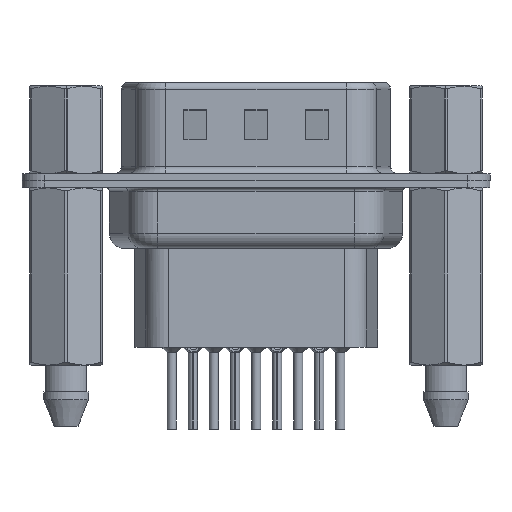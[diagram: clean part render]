
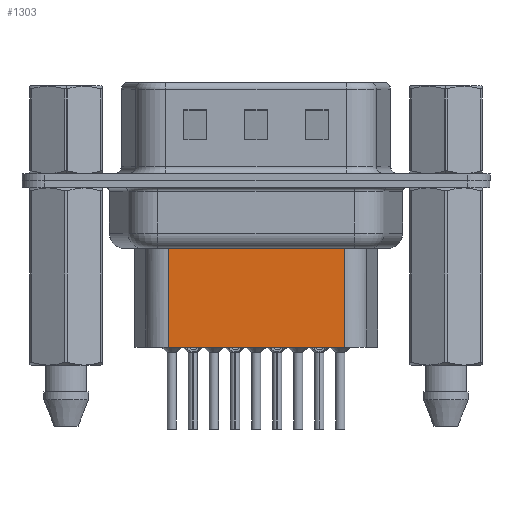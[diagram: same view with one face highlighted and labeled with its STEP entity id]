
A CAD part, front view. The second image highlights one B-rep face of the part: STEP entity #1303.
In plain terms, the highlighted planar face has unit normal (0, -1, 0).
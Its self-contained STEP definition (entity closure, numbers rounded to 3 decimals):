
#412 = DIRECTION ( 'NONE',  ( -1., 0., 0. ) ) ;
#484 = LINE ( 'NONE', #8656, #5251 ) ;
#1233 = VECTOR ( 'NONE', #412, 1000. ) ;
#1303 = ADVANCED_FACE ( 'NONE', ( #20888 ), #2808, .T. ) ;
#1419 = AXIS2_PLACEMENT_3D ( 'NONE', #17182, #10884, #6892 ) ;
#1904 = VECTOR ( 'NONE', #1964, 1000. ) ;
#1964 = DIRECTION ( 'NONE',  ( 0., 0., -1. ) ) ;
#2642 = VERTEX_POINT ( 'NONE', #18498 ) ;
#2776 = ORIENTED_EDGE ( 'NONE', *, *, #24345, .T. ) ;
#2808 = PLANE ( 'NONE',  #1419 ) ;
#3517 = LINE ( 'NONE', #9584, #23152 ) ;
#4767 = ORIENTED_EDGE ( 'NONE', *, *, #11726, .F. ) ;
#5251 = VECTOR ( 'NONE', #14595, 1000. ) ;
#5622 = DIRECTION ( 'NONE',  ( -1., 0., 0. ) ) ;
#6504 = EDGE_LOOP ( 'NONE', ( #4767, #2776, #11602, #25005 ) ) ;
#6892 = DIRECTION ( 'NONE',  ( 1., 0., 0. ) ) ;
#6987 = LINE ( 'NONE', #18492, #1233 ) ;
#7474 = VERTEX_POINT ( 'NONE', #15951 ) ;
#7946 = VERTEX_POINT ( 'NONE', #21396 ) ;
#8275 = CARTESIAN_POINT ( 'NONE',  ( 6.706, -3.5, -10.95 ) ) ;
#8656 = CARTESIAN_POINT ( 'NONE',  ( 6.706, -3.5, -3.1 ) ) ;
#9584 = CARTESIAN_POINT ( 'NONE',  ( 6.459, -3.5, -4.097 ) ) ;
#10884 = DIRECTION ( 'NONE',  ( 0., -1., 0. ) ) ;
#10988 = EDGE_CURVE ( 'NONE', #2642, #19853, #484, .T. ) ;
#11602 = ORIENTED_EDGE ( 'NONE', *, *, #10988, .T. ) ;
#11726 = EDGE_CURVE ( 'NONE', #7474, #7946, #25851, .T. ) ;
#14595 = DIRECTION ( 'NONE',  ( 0., 0., -1. ) ) ;
#15951 = CARTESIAN_POINT ( 'NONE',  ( 18.294, -3.5, -4.097 ) ) ;
#17182 = CARTESIAN_POINT ( 'NONE',  ( 6.706, -3.5, -3.1 ) ) ;
#18492 = CARTESIAN_POINT ( 'NONE',  ( 6.706, -3.5, -10.95 ) ) ;
#18498 = CARTESIAN_POINT ( 'NONE',  ( 6.706, -3.5, -4.097 ) ) ;
#19853 = VERTEX_POINT ( 'NONE', #8275 ) ;
#20888 = FACE_OUTER_BOUND ( 'NONE', #6504, .T. ) ;
#21396 = CARTESIAN_POINT ( 'NONE',  ( 18.294, -3.5, -10.95 ) ) ;
#23152 = VECTOR ( 'NONE', #5622, 1000. ) ;
#23870 = CARTESIAN_POINT ( 'NONE',  ( 18.294, -3.5, -3.1 ) ) ;
#24345 = EDGE_CURVE ( 'NONE', #7474, #2642, #3517, .T. ) ;
#25005 = ORIENTED_EDGE ( 'NONE', *, *, #25266, .F. ) ;
#25266 = EDGE_CURVE ( 'NONE', #7946, #19853, #6987, .T. ) ;
#25851 = LINE ( 'NONE', #23870, #1904 ) ;
